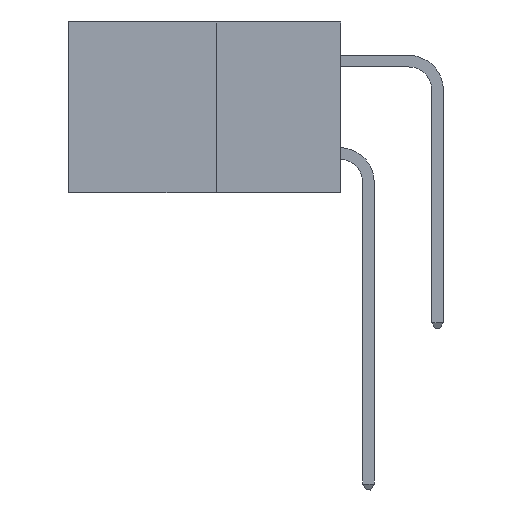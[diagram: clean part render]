
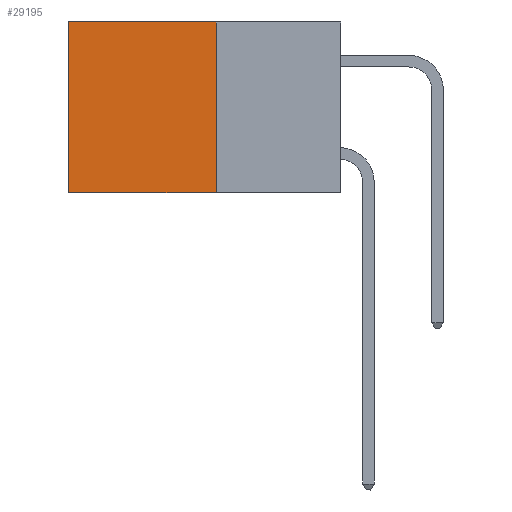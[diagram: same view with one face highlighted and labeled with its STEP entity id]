
A CAD part, left-side view. The second image highlights one B-rep face of the part: STEP entity #29195.
In plain terms, the highlighted planar face has unit normal (-1, 0, 0).
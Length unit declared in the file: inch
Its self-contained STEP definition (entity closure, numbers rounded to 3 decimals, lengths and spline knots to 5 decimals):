
#1878 = CARTESIAN_POINT ( 'NONE',  ( 0.277, 0.27, -0.37 ) ) ;
#1987 = DIRECTION ( 'NONE',  ( 0., 0., -1. ) ) ;
#2003 = DIRECTION ( 'NONE',  ( 0., 0., -1. ) ) ;
#3469 = LINE ( 'NONE', #19393, #20896 ) ;
#3625 = VERTEX_POINT ( 'NONE', #20156 ) ;
#6263 = LINE ( 'NONE', #12501, #29291 ) ;
#6454 = DIRECTION ( 'NONE',  ( 0., 1., 0. ) ) ;
#7507 = VERTEX_POINT ( 'NONE', #24610 ) ;
#8471 = EDGE_CURVE ( 'NONE', #7507, #3625, #17830, .T. ) ;
#10722 = ORIENTED_EDGE ( 'NONE', *, *, #8471, .T. ) ;
#10734 = VECTOR ( 'NONE', #6454, 39.37008 ) ;
#12501 = CARTESIAN_POINT ( 'NONE',  ( 0.277, 0.27, -0.37 ) ) ;
#12527 = CARTESIAN_POINT ( 'NONE',  ( 0.277, 0.59, -0.37 ) ) ;
#13192 = EDGE_CURVE ( 'NONE', #7507, #18315, #3469, .T. ) ;
#13785 = CARTESIAN_POINT ( 'NONE',  ( 0.277, 0.59, -0.37 ) ) ;
#14636 = CARTESIAN_POINT ( 'NONE',  ( 0.277, 0.27, -0.37 ) ) ;
#16174 = DIRECTION ( 'NONE',  ( 1., 0., 0. ) ) ;
#16250 = LINE ( 'NONE', #13785, #21825 ) ;
#16688 = ORIENTED_EDGE ( 'NONE', *, *, #23290, .T. ) ;
#17830 = LINE ( 'NONE', #23067, #10734 ) ;
#18315 = VERTEX_POINT ( 'NONE', #14636 ) ;
#18421 = VERTEX_POINT ( 'NONE', #12527 ) ;
#19393 = CARTESIAN_POINT ( 'NONE',  ( 0.277, 0.27, -0.37 ) ) ;
#20156 = CARTESIAN_POINT ( 'NONE',  ( 0.277, 0.59, 0. ) ) ;
#20256 = EDGE_LOOP ( 'NONE', ( #16688, #26186, #27994, #10722 ) ) ;
#20896 = VECTOR ( 'NONE', #21743, 39.37008 ) ;
#21743 = DIRECTION ( 'NONE',  ( 0., 0., -1. ) ) ;
#21825 = VECTOR ( 'NONE', #2003, 39.37008 ) ;
#23067 = CARTESIAN_POINT ( 'NONE',  ( 0.277, 0.27, 0. ) ) ;
#23290 = EDGE_CURVE ( 'NONE', #3625, #18421, #16250, .T. ) ;
#24610 = CARTESIAN_POINT ( 'NONE',  ( 0.277, 0.27, 0. ) ) ;
#26186 = ORIENTED_EDGE ( 'NONE', *, *, #29521, .F. ) ;
#26397 = FACE_OUTER_BOUND ( 'NONE', #20256, .T. ) ;
#26788 = DIRECTION ( 'NONE',  ( 0., 1., 0. ) ) ;
#27994 = ORIENTED_EDGE ( 'NONE', *, *, #13192, .F. ) ;
#29195 = ADVANCED_FACE ( 'NONE', ( #26397 ), #30379, .F. ) ;
#29291 = VECTOR ( 'NONE', #26788, 39.37008 ) ;
#29521 = EDGE_CURVE ( 'NONE', #18315, #18421, #6263, .T. ) ;
#30217 = AXIS2_PLACEMENT_3D ( 'NONE', #1878, #16174, #1987 ) ;
#30379 = PLANE ( 'NONE',  #30217 ) ;
